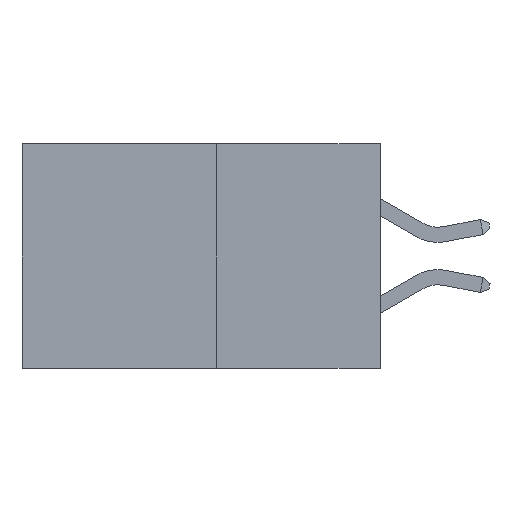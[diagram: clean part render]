
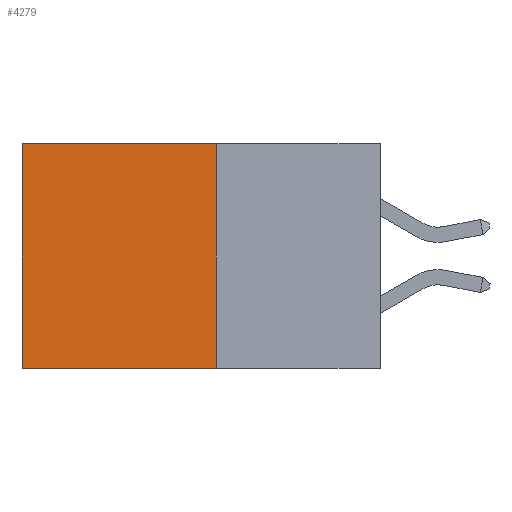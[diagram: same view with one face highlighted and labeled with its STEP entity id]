
A CAD part, left-side view. The second image highlights one B-rep face of the part: STEP entity #4279.
In plain terms, the highlighted planar face has unit normal (-1, 0, 0).
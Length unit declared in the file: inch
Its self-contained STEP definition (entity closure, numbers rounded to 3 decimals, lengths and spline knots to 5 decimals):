
#872 = CARTESIAN_POINT ( 'NONE',  ( 0.277, 0.59, -0.37 ) ) ;
#1199 = DIRECTION ( 'NONE',  ( 0., 1., 0. ) ) ;
#1509 = FACE_OUTER_BOUND ( 'NONE', #2745, .T. ) ;
#2101 = CARTESIAN_POINT ( 'NONE',  ( 0.277, 0.27, -0.37 ) ) ;
#2745 = EDGE_LOOP ( 'NONE', ( #4904, #23180, #14259, #20598 ) ) ;
#3377 = CARTESIAN_POINT ( 'NONE',  ( 0.277, 0.27, 0. ) ) ;
#3741 = DIRECTION ( 'NONE',  ( 0., 0., -1. ) ) ;
#3770 = DIRECTION ( 'NONE',  ( 1., 0., 0. ) ) ;
#3844 = VECTOR ( 'NONE', #23404, 39.37008 ) ;
#3867 = CARTESIAN_POINT ( 'NONE',  ( 0.277, 0.27, -0.37 ) ) ;
#4118 = PLANE ( 'NONE',  #13780 ) ;
#4279 = ADVANCED_FACE ( 'NONE', ( #1509 ), #4118, .F. ) ;
#4904 = ORIENTED_EDGE ( 'NONE', *, *, #13193, .T. ) ;
#5996 = CARTESIAN_POINT ( 'NONE',  ( 0.277, 0.59, -0.37 ) ) ;
#7904 = VERTEX_POINT ( 'NONE', #2101 ) ;
#8813 = VECTOR ( 'NONE', #11739, 39.37008 ) ;
#9161 = EDGE_CURVE ( 'NONE', #12079, #7904, #17776, .T. ) ;
#9397 = VECTOR ( 'NONE', #11592, 39.37008 ) ;
#9635 = VERTEX_POINT ( 'NONE', #21168 ) ;
#9808 = CARTESIAN_POINT ( 'NONE',  ( 0.277, 0.27, 0. ) ) ;
#10687 = CARTESIAN_POINT ( 'NONE',  ( 0.277, 0.27, -0.37 ) ) ;
#11136 = VECTOR ( 'NONE', #1199, 39.37008 ) ;
#11592 = DIRECTION ( 'NONE',  ( 0., 1., 0. ) ) ;
#11691 = LINE ( 'NONE', #17501, #11136 ) ;
#11739 = DIRECTION ( 'NONE',  ( 0., 0., -1. ) ) ;
#12079 = VERTEX_POINT ( 'NONE', #3377 ) ;
#13160 = EDGE_CURVE ( 'NONE', #12079, #9635, #18582, .T. ) ;
#13193 = EDGE_CURVE ( 'NONE', #9635, #19547, #13715, .T. ) ;
#13715 = LINE ( 'NONE', #872, #8813 ) ;
#13780 = AXIS2_PLACEMENT_3D ( 'NONE', #3867, #3770, #3741 ) ;
#14259 = ORIENTED_EDGE ( 'NONE', *, *, #9161, .F. ) ;
#17501 = CARTESIAN_POINT ( 'NONE',  ( 0.277, 0.27, -0.37 ) ) ;
#17776 = LINE ( 'NONE', #10687, #3844 ) ;
#18582 = LINE ( 'NONE', #9808, #9397 ) ;
#19547 = VERTEX_POINT ( 'NONE', #5996 ) ;
#20243 = EDGE_CURVE ( 'NONE', #7904, #19547, #11691, .T. ) ;
#20598 = ORIENTED_EDGE ( 'NONE', *, *, #13160, .T. ) ;
#21168 = CARTESIAN_POINT ( 'NONE',  ( 0.277, 0.59, 0. ) ) ;
#23180 = ORIENTED_EDGE ( 'NONE', *, *, #20243, .F. ) ;
#23404 = DIRECTION ( 'NONE',  ( 0., 0., -1. ) ) ;
